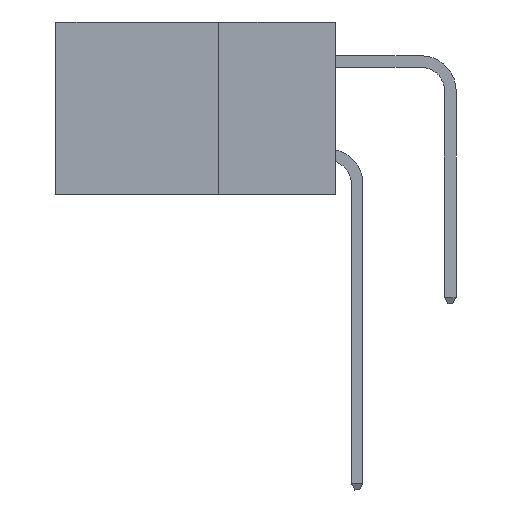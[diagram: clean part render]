
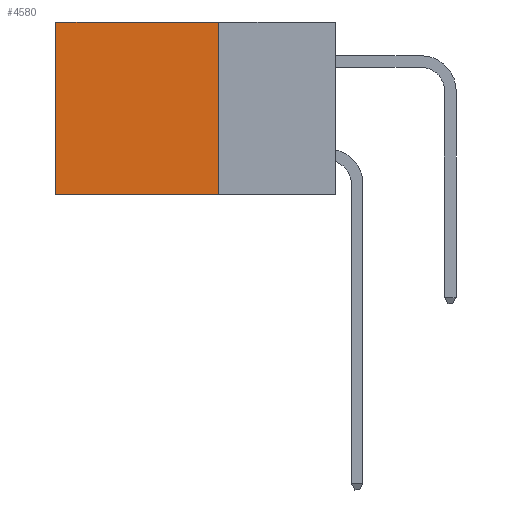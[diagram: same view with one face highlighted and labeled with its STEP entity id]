
A CAD part, left-side view. The second image highlights one B-rep face of the part: STEP entity #4580.
In plain terms, the highlighted planar face has unit normal (-1, 0, 0).
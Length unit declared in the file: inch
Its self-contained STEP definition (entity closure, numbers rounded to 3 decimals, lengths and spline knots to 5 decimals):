
#656 = PLANE ( 'NONE',  #13744 ) ;
#1020 = DIRECTION ( 'NONE',  ( 0., 0., -1. ) ) ;
#2535 = VECTOR ( 'NONE', #1020, 39.37008 ) ;
#3184 = DIRECTION ( 'NONE',  ( 0., 0., -1. ) ) ;
#3380 = ORIENTED_EDGE ( 'NONE', *, *, #16402, .T. ) ;
#3412 = LINE ( 'NONE', #3787, #5958 ) ;
#3787 = CARTESIAN_POINT ( 'NONE',  ( 0.2875, 0.25, -0.37 ) ) ;
#4122 = VERTEX_POINT ( 'NONE', #11281 ) ;
#4339 = VECTOR ( 'NONE', #5378, 39.37008 ) ;
#4423 = FACE_OUTER_BOUND ( 'NONE', #14603, .T. ) ;
#4580 = ADVANCED_FACE ( 'NONE', ( #4423 ), #656, .F. ) ;
#4782 = VECTOR ( 'NONE', #3184, 39.37008 ) ;
#5039 = VERTEX_POINT ( 'NONE', #16002 ) ;
#5327 = LINE ( 'NONE', #12955, #4339 ) ;
#5378 = DIRECTION ( 'NONE',  ( 0., 1., 0. ) ) ;
#5834 = DIRECTION ( 'NONE',  ( 1., 0., 0. ) ) ;
#5958 = VECTOR ( 'NONE', #10162, 39.37008 ) ;
#6121 = VERTEX_POINT ( 'NONE', #14630 ) ;
#6954 = CARTESIAN_POINT ( 'NONE',  ( 0.2875, 0.25, -0.37 ) ) ;
#7903 = ORIENTED_EDGE ( 'NONE', *, *, #11479, .F. ) ;
#8338 = CARTESIAN_POINT ( 'NONE',  ( 0.2875, 0.6, 0. ) ) ;
#8349 = VERTEX_POINT ( 'NONE', #6954 ) ;
#8686 = EDGE_CURVE ( 'NONE', #8349, #6121, #3412, .T. ) ;
#8944 = EDGE_CURVE ( 'NONE', #4122, #6121, #16115, .T. ) ;
#10162 = DIRECTION ( 'NONE',  ( 0., 1., 0. ) ) ;
#11281 = CARTESIAN_POINT ( 'NONE',  ( 0.2875, 0.6, 0. ) ) ;
#11479 = EDGE_CURVE ( 'NONE', #5039, #8349, #14422, .T. ) ;
#11925 = ORIENTED_EDGE ( 'NONE', *, *, #8944, .T. ) ;
#12955 = CARTESIAN_POINT ( 'NONE',  ( 0.2875, 0.25, 0. ) ) ;
#13256 = CARTESIAN_POINT ( 'NONE',  ( 0.2875, 0.25, 0. ) ) ;
#13348 = DIRECTION ( 'NONE',  ( 0., 0., -1. ) ) ;
#13552 = ORIENTED_EDGE ( 'NONE', *, *, #8686, .F. ) ;
#13561 = CARTESIAN_POINT ( 'NONE',  ( 0.2875, 0.25, 0. ) ) ;
#13744 = AXIS2_PLACEMENT_3D ( 'NONE', #13256, #5834, #13348 ) ;
#14422 = LINE ( 'NONE', #13561, #2535 ) ;
#14603 = EDGE_LOOP ( 'NONE', ( #11925, #13552, #7903, #3380 ) ) ;
#14630 = CARTESIAN_POINT ( 'NONE',  ( 0.2875, 0.6, -0.37 ) ) ;
#16002 = CARTESIAN_POINT ( 'NONE',  ( 0.2875, 0.25, 0. ) ) ;
#16115 = LINE ( 'NONE', #8338, #4782 ) ;
#16402 = EDGE_CURVE ( 'NONE', #5039, #4122, #5327, .T. ) ;
